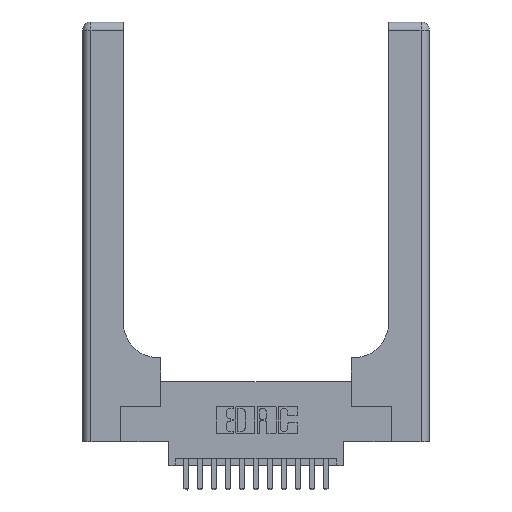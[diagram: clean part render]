
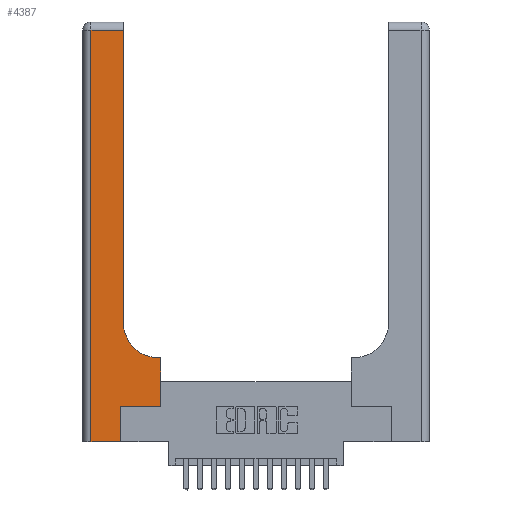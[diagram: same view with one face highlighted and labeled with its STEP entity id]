
A CAD part, top view. The second image highlights one B-rep face of the part: STEP entity #4387.
In plain terms, the highlighted planar face has unit normal (0, 0, 1).
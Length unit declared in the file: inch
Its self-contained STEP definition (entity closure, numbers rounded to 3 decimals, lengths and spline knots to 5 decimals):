
#51 = VERTEX_POINT ( 'NONE', #3993 ) ;
#78 = EDGE_CURVE ( 'NONE', #51, #14999, #5093, .T. ) ;
#79 = VERTEX_POINT ( 'NONE', #13927 ) ;
#99 = DIRECTION ( 'NONE',  ( -1., 0., 0. ) ) ;
#103 = EDGE_CURVE ( 'NONE', #16891, #15019, #7509, .T. ) ;
#166 = DIRECTION ( 'NONE',  ( 0., 1., 0. ) ) ;
#497 = CARTESIAN_POINT ( 'NONE',  ( 0.06, 2.94, 0.37 ) ) ;
#547 = DIRECTION ( 'NONE',  ( 0., -1., 0. ) ) ;
#836 = ORIENTED_EDGE ( 'NONE', *, *, #2448, .T. ) ;
#1215 = CARTESIAN_POINT ( 'NONE',  ( 0.269, 0., 0.37 ) ) ;
#1631 = DIRECTION ( 'NONE',  ( 1., 0., 0. ) ) ;
#1993 = VECTOR ( 'NONE', #547, 39.37008 ) ;
#2006 = DIRECTION ( 'NONE',  ( -1., 0., 0. ) ) ;
#2109 = VECTOR ( 'NONE', #5553, 39.37008 ) ;
#2413 = DIRECTION ( 'NONE',  ( -1., 0., 0. ) ) ;
#2448 = EDGE_CURVE ( 'NONE', #79, #14742, #16024, .T. ) ;
#2726 = VECTOR ( 'NONE', #13120, 39.37008 ) ;
#3210 = CARTESIAN_POINT ( 'NONE',  ( 0.2915, 3., 0.37 ) ) ;
#3358 = CARTESIAN_POINT ( 'NONE',  ( 0., 3., 0.37 ) ) ;
#3412 = DIRECTION ( 'NONE',  ( 1., 0., 0. ) ) ;
#3831 = ORIENTED_EDGE ( 'NONE', *, *, #17596, .T. ) ;
#3993 = CARTESIAN_POINT ( 'NONE',  ( 0.269, 0., 0.37 ) ) ;
#4228 = CARTESIAN_POINT ( 'NONE',  ( 0.5585, 0.25, 0.37 ) ) ;
#4270 = FACE_OUTER_BOUND ( 'NONE', #7284, .T. ) ;
#4387 = ADVANCED_FACE ( 'NONE', ( #4270 ), #6099, .F. ) ;
#4401 = VECTOR ( 'NONE', #6840, 39.37008 ) ;
#4724 = EDGE_CURVE ( 'NONE', #14742, #16891, #6495, .T. ) ;
#5093 = LINE ( 'NONE', #1215, #4401 ) ;
#5493 = AXIS2_PLACEMENT_3D ( 'NONE', #12798, #15647, #3412 ) ;
#5553 = DIRECTION ( 'NONE',  ( 1., 0., 0. ) ) ;
#5739 = VECTOR ( 'NONE', #99, 39.37008 ) ;
#6099 = PLANE ( 'NONE',  #18067 ) ;
#6105 = CARTESIAN_POINT ( 'NONE',  ( 0.06, 3., 0.37 ) ) ;
#6241 = VERTEX_POINT ( 'NONE', #15881 ) ;
#6323 = LINE ( 'NONE', #9762, #2109 ) ;
#6495 = LINE ( 'NONE', #3210, #2726 ) ;
#6840 = DIRECTION ( 'NONE',  ( 0., 1., 0. ) ) ;
#7219 = LINE ( 'NONE', #4228, #10721 ) ;
#7284 = EDGE_LOOP ( 'NONE', ( #16856, #17752, #12928, #9519, #10462, #17361, #16073, #3831, #836 ) ) ;
#7297 = CARTESIAN_POINT ( 'NONE',  ( 0.5585, 0.25, 0.37 ) ) ;
#7451 = VECTOR ( 'NONE', #1631, 39.37008 ) ;
#7509 = LINE ( 'NONE', #15582, #5739 ) ;
#8181 = CARTESIAN_POINT ( 'NONE',  ( 0.5585, 0.6, 0.37 ) ) ;
#8719 = CARTESIAN_POINT ( 'NONE',  ( 0.269, 0.25, 0.37 ) ) ;
#8812 = CARTESIAN_POINT ( 'NONE',  ( 0.2915, 2.94, 0.37 ) ) ;
#9257 = LINE ( 'NONE', #6105, #1993 ) ;
#9442 = EDGE_CURVE ( 'NONE', #15019, #6241, #9257, .T. ) ;
#9519 = ORIENTED_EDGE ( 'NONE', *, *, #12345, .T. ) ;
#9762 = CARTESIAN_POINT ( 'NONE',  ( 0.269, 0.25, 0.37 ) ) ;
#10407 = VECTOR ( 'NONE', #2413, 39.37008 ) ;
#10462 = ORIENTED_EDGE ( 'NONE', *, *, #78, .T. ) ;
#10721 = VECTOR ( 'NONE', #166, 39.37008 ) ;
#12243 = CARTESIAN_POINT ( 'NONE',  ( 0.2915, 0.85, 0.37 ) ) ;
#12345 = EDGE_CURVE ( 'NONE', #6241, #51, #13144, .T. ) ;
#12359 = EDGE_CURVE ( 'NONE', #17296, #17722, #7219, .T. ) ;
#12798 = CARTESIAN_POINT ( 'NONE',  ( 0.5415, 0.85, 0.37 ) ) ;
#12928 = ORIENTED_EDGE ( 'NONE', *, *, #9442, .T. ) ;
#13120 = DIRECTION ( 'NONE',  ( 0., 1., 0. ) ) ;
#13144 = LINE ( 'NONE', #14287, #7451 ) ;
#13145 = DIRECTION ( 'NONE',  ( 0., 0., -1. ) ) ;
#13618 = CARTESIAN_POINT ( 'NONE',  ( 0.2915, 0.6, 0.37 ) ) ;
#13927 = CARTESIAN_POINT ( 'NONE',  ( 0.5415, 0.6, 0.37 ) ) ;
#14287 = CARTESIAN_POINT ( 'NONE',  ( 0., 0., 0.37 ) ) ;
#14742 = VERTEX_POINT ( 'NONE', #12243 ) ;
#14999 = VERTEX_POINT ( 'NONE', #8719 ) ;
#15019 = VERTEX_POINT ( 'NONE', #497 ) ;
#15480 = EDGE_CURVE ( 'NONE', #14999, #17296, #6323, .T. ) ;
#15582 = CARTESIAN_POINT ( 'NONE',  ( 0., 2.94, 0.37 ) ) ;
#15647 = DIRECTION ( 'NONE',  ( 0., 0., -1. ) ) ;
#15881 = CARTESIAN_POINT ( 'NONE',  ( 0.06, 0., 0.37 ) ) ;
#16024 = CIRCLE ( 'NONE', #5493, 0.25 ) ;
#16073 = ORIENTED_EDGE ( 'NONE', *, *, #12359, .T. ) ;
#16856 = ORIENTED_EDGE ( 'NONE', *, *, #4724, .T. ) ;
#16891 = VERTEX_POINT ( 'NONE', #8812 ) ;
#17288 = LINE ( 'NONE', #13618, #10407 ) ;
#17296 = VERTEX_POINT ( 'NONE', #7297 ) ;
#17361 = ORIENTED_EDGE ( 'NONE', *, *, #15480, .T. ) ;
#17596 = EDGE_CURVE ( 'NONE', #17722, #79, #17288, .T. ) ;
#17722 = VERTEX_POINT ( 'NONE', #8181 ) ;
#17752 = ORIENTED_EDGE ( 'NONE', *, *, #103, .T. ) ;
#18067 = AXIS2_PLACEMENT_3D ( 'NONE', #3358, #13145, #2006 ) ;
